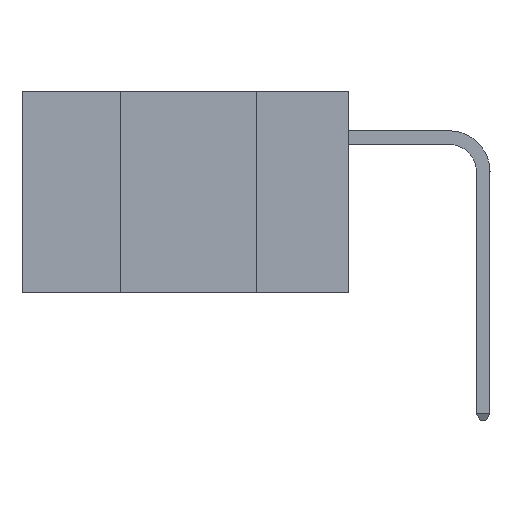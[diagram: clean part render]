
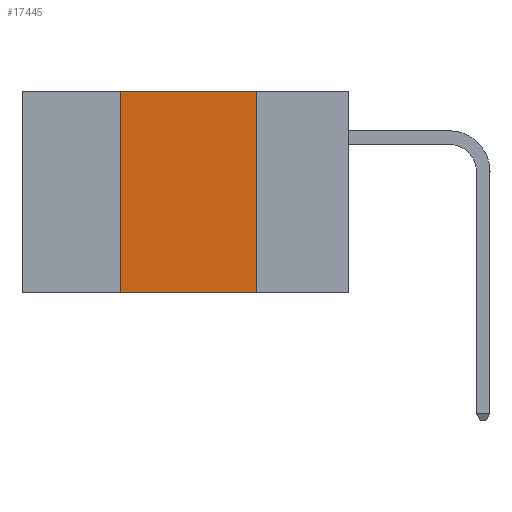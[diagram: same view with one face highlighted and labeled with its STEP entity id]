
A CAD part, left-side view. The second image highlights one B-rep face of the part: STEP entity #17445.
In plain terms, the highlighted planar face has unit normal (-1, 0, 0).
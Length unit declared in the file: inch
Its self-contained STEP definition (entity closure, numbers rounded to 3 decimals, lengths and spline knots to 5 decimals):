
#2265 = EDGE_CURVE ( 'NONE', #35905, #16572, #19756, .T. ) ;
#2319 = EDGE_CURVE ( 'NONE', #4842, #16572, #17962, .T. ) ;
#3238 = EDGE_LOOP ( 'NONE', ( #15216, #29211, #35501, #22679 ) ) ;
#3319 = CARTESIAN_POINT ( 'NONE',  ( 0., 0.6, 0. ) ) ;
#4613 = CARTESIAN_POINT ( 'NONE',  ( 0., 0.17, 0. ) ) ;
#4842 = VERTEX_POINT ( 'NONE', #35644 ) ;
#4844 = CARTESIAN_POINT ( 'NONE',  ( 0., 0.17, 0. ) ) ;
#4961 = CARTESIAN_POINT ( 'NONE',  ( 0., 0.6, -0.37 ) ) ;
#4984 = LINE ( 'NONE', #3319, #25962 ) ;
#7509 = FACE_OUTER_BOUND ( 'NONE', #3238, .T. ) ;
#7902 = AXIS2_PLACEMENT_3D ( 'NONE', #28380, #11402, #31166 ) ;
#11402 = DIRECTION ( 'NONE',  ( 1., 0., 0. ) ) ;
#12199 = VECTOR ( 'NONE', #24796, 39.37008 ) ;
#12843 = VERTEX_POINT ( 'NONE', #19159 ) ;
#14149 = DIRECTION ( 'NONE',  ( 0., 0., 1. ) ) ;
#15216 = ORIENTED_EDGE ( 'NONE', *, *, #2265, .F. ) ;
#16572 = VERTEX_POINT ( 'NONE', #35207 ) ;
#17445 = ADVANCED_FACE ( 'NONE', ( #7509 ), #22723, .F. ) ;
#17504 = VECTOR ( 'NONE', #14149, 39.37008 ) ;
#17962 = LINE ( 'NONE', #4961, #32081 ) ;
#19159 = CARTESIAN_POINT ( 'NONE',  ( 0., 0.42, 0. ) ) ;
#19756 = LINE ( 'NONE', #4844, #12199 ) ;
#22679 = ORIENTED_EDGE ( 'NONE', *, *, #2319, .T. ) ;
#22723 = PLANE ( 'NONE',  #7902 ) ;
#22767 = CARTESIAN_POINT ( 'NONE',  ( 0., 0.42, 0. ) ) ;
#24796 = DIRECTION ( 'NONE',  ( 0., 0., -1. ) ) ;
#25962 = VECTOR ( 'NONE', #31865, 39.37008 ) ;
#28380 = CARTESIAN_POINT ( 'NONE',  ( 0., 0.6, 0. ) ) ;
#28468 = EDGE_CURVE ( 'NONE', #4842, #12843, #32496, .T. ) ;
#29211 = ORIENTED_EDGE ( 'NONE', *, *, #36304, .F. ) ;
#30539 = DIRECTION ( 'NONE',  ( 0., -1., 0. ) ) ;
#31166 = DIRECTION ( 'NONE',  ( 0., 0., -1. ) ) ;
#31865 = DIRECTION ( 'NONE',  ( 0., -1., 0. ) ) ;
#32081 = VECTOR ( 'NONE', #30539, 39.37008 ) ;
#32496 = LINE ( 'NONE', #22767, #17504 ) ;
#35207 = CARTESIAN_POINT ( 'NONE',  ( 0., 0.17, -0.37 ) ) ;
#35501 = ORIENTED_EDGE ( 'NONE', *, *, #28468, .F. ) ;
#35644 = CARTESIAN_POINT ( 'NONE',  ( 0., 0.42, -0.37 ) ) ;
#35905 = VERTEX_POINT ( 'NONE', #4613 ) ;
#36304 = EDGE_CURVE ( 'NONE', #12843, #35905, #4984, .T. ) ;
